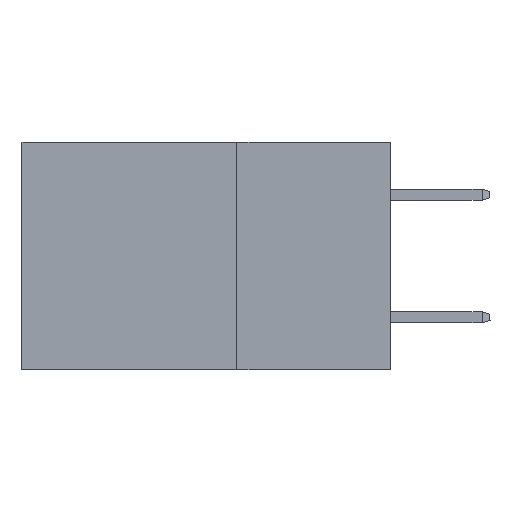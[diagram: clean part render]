
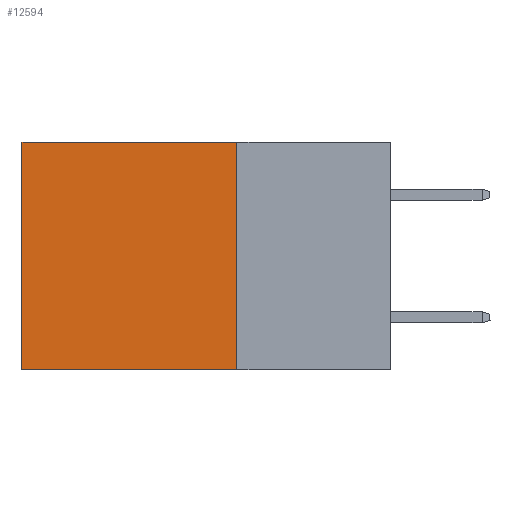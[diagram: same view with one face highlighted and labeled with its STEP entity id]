
A CAD part, left-side view. The second image highlights one B-rep face of the part: STEP entity #12594.
In plain terms, the highlighted planar face has unit normal (-1, 0, 0).
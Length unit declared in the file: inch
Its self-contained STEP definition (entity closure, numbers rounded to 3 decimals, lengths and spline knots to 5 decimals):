
#2595 = CARTESIAN_POINT ( 'NONE',  ( 0.2875, 0.25, -0.37 ) ) ;
#2650 = VECTOR ( 'NONE', #8465, 39.37008 ) ;
#3020 = VERTEX_POINT ( 'NONE', #7533 ) ;
#4692 = EDGE_CURVE ( 'NONE', #7956, #3020, #5146, .T. ) ;
#5146 = LINE ( 'NONE', #17042, #14840 ) ;
#5188 = CARTESIAN_POINT ( 'NONE',  ( 0.2875, 0.25, -0.37 ) ) ;
#5303 = CARTESIAN_POINT ( 'NONE',  ( 0.2875, 0.6, 0. ) ) ;
#7533 = CARTESIAN_POINT ( 'NONE',  ( 0.2875, 0.6, -0.37 ) ) ;
#7750 = EDGE_CURVE ( 'NONE', #20263, #7956, #18794, .T. ) ;
#7956 = VERTEX_POINT ( 'NONE', #5303 ) ;
#8249 = ORIENTED_EDGE ( 'NONE', *, *, #7750, .T. ) ;
#8345 = DIRECTION ( 'NONE',  ( 0., 0., -1. ) ) ;
#8465 = DIRECTION ( 'NONE',  ( 0., 1., 0. ) ) ;
#8569 = LINE ( 'NONE', #15500, #16434 ) ;
#8929 = DIRECTION ( 'NONE',  ( 0., 0., -1. ) ) ;
#9421 = EDGE_CURVE ( 'NONE', #19156, #3020, #9851, .T. ) ;
#9851 = LINE ( 'NONE', #2595, #21515 ) ;
#10873 = ORIENTED_EDGE ( 'NONE', *, *, #9421, .F. ) ;
#12594 = ADVANCED_FACE ( 'NONE', ( #20977 ), #19363, .F. ) ;
#13550 = DIRECTION ( 'NONE',  ( 0., 0., -1. ) ) ;
#13930 = CARTESIAN_POINT ( 'NONE',  ( 0.2875, 0.25, 0. ) ) ;
#14840 = VECTOR ( 'NONE', #13550, 39.37008 ) ;
#15500 = CARTESIAN_POINT ( 'NONE',  ( 0.2875, 0.25, 0. ) ) ;
#15961 = ORIENTED_EDGE ( 'NONE', *, *, #4692, .T. ) ;
#16434 = VECTOR ( 'NONE', #8345, 39.37008 ) ;
#16683 = ORIENTED_EDGE ( 'NONE', *, *, #16847, .F. ) ;
#16847 = EDGE_CURVE ( 'NONE', #20263, #19156, #8569, .T. ) ;
#17042 = CARTESIAN_POINT ( 'NONE',  ( 0.2875, 0.6, 0. ) ) ;
#18453 = CARTESIAN_POINT ( 'NONE',  ( 0.2875, 0.25, 0. ) ) ;
#18794 = LINE ( 'NONE', #18453, #2650 ) ;
#18901 = AXIS2_PLACEMENT_3D ( 'NONE', #13930, #21079, #8929 ) ;
#19156 = VERTEX_POINT ( 'NONE', #5188 ) ;
#19363 = PLANE ( 'NONE',  #18901 ) ;
#20263 = VERTEX_POINT ( 'NONE', #20277 ) ;
#20277 = CARTESIAN_POINT ( 'NONE',  ( 0.2875, 0.25, 0. ) ) ;
#20977 = FACE_OUTER_BOUND ( 'NONE', #21057, .T. ) ;
#21057 = EDGE_LOOP ( 'NONE', ( #15961, #10873, #16683, #8249 ) ) ;
#21079 = DIRECTION ( 'NONE',  ( 1., 0., 0. ) ) ;
#21515 = VECTOR ( 'NONE', #21998, 39.37008 ) ;
#21998 = DIRECTION ( 'NONE',  ( 0., 1., 0. ) ) ;
